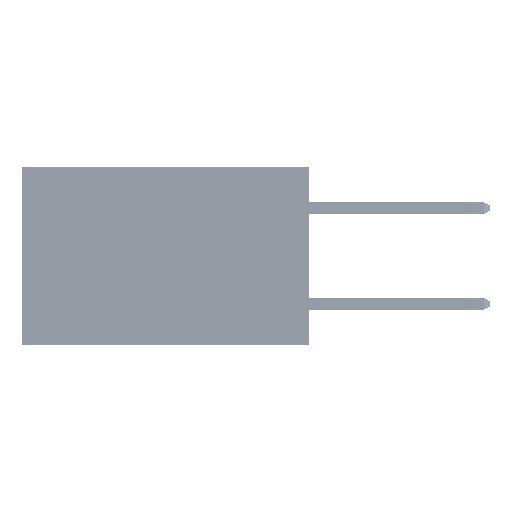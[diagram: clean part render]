
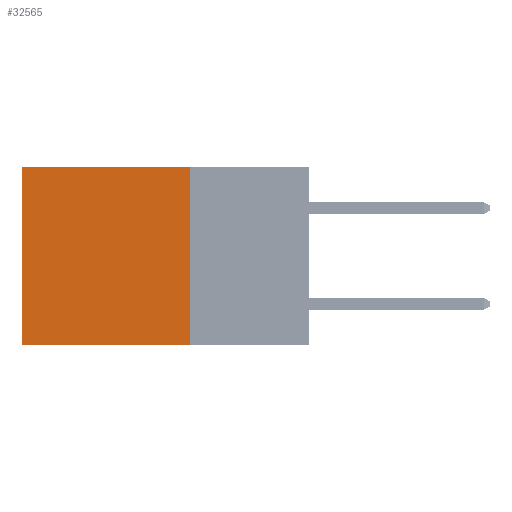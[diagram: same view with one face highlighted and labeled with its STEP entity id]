
A CAD part, left-side view. The second image highlights one B-rep face of the part: STEP entity #32565.
In plain terms, the highlighted planar face has unit normal (-1, 0, 0).
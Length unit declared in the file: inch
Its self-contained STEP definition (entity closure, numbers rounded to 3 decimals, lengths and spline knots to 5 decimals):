
#856 = PLANE ( 'NONE',  #13473 ) ;
#861 = CARTESIAN_POINT ( 'NONE',  ( 0.2875, 0.25, -0.37 ) ) ;
#1019 = ORIENTED_EDGE ( 'NONE', *, *, #51578, .T. ) ;
#1751 = CARTESIAN_POINT ( 'NONE',  ( 0.2875, 0.25, 0. ) ) ;
#2517 = VECTOR ( 'NONE', #15506, 39.37008 ) ;
#5125 = VECTOR ( 'NONE', #17125, 39.37008 ) ;
#6104 = DIRECTION ( 'NONE',  ( 0., 1., 0. ) ) ;
#7245 = EDGE_LOOP ( 'NONE', ( #50774, #39145, #17629, #1019 ) ) ;
#7819 = EDGE_CURVE ( 'NONE', #8032, #37418, #15131, .T. ) ;
#8032 = VERTEX_POINT ( 'NONE', #20796 ) ;
#10239 = VECTOR ( 'NONE', #6104, 39.37008 ) ;
#10594 = CARTESIAN_POINT ( 'NONE',  ( 0.2875, 0.25, -0.37 ) ) ;
#12822 = CARTESIAN_POINT ( 'NONE',  ( 0.2875, 0.25, 0. ) ) ;
#13473 = AXIS2_PLACEMENT_3D ( 'NONE', #21171, #41553, #17296 ) ;
#15131 = LINE ( 'NONE', #39754, #2517 ) ;
#15506 = DIRECTION ( 'NONE',  ( 0., 0., -1. ) ) ;
#15792 = LINE ( 'NONE', #1751, #28513 ) ;
#17125 = DIRECTION ( 'NONE',  ( 0., 1., 0. ) ) ;
#17296 = DIRECTION ( 'NONE',  ( 0., 0., -1. ) ) ;
#17629 = ORIENTED_EDGE ( 'NONE', *, *, #23222, .F. ) ;
#20382 = LINE ( 'NONE', #29794, #10239 ) ;
#20796 = CARTESIAN_POINT ( 'NONE',  ( 0.2875, 0.6, 0. ) ) ;
#21171 = CARTESIAN_POINT ( 'NONE',  ( 0.2875, 0.25, 0. ) ) ;
#23222 = EDGE_CURVE ( 'NONE', #39502, #45514, #15792, .T. ) ;
#26594 = LINE ( 'NONE', #861, #5125 ) ;
#28513 = VECTOR ( 'NONE', #30048, 39.37008 ) ;
#29794 = CARTESIAN_POINT ( 'NONE',  ( 0.2875, 0.25, 0. ) ) ;
#30048 = DIRECTION ( 'NONE',  ( 0., 0., -1. ) ) ;
#32565 = ADVANCED_FACE ( 'NONE', ( #36219 ), #856, .F. ) ;
#36219 = FACE_OUTER_BOUND ( 'NONE', #7245, .T. ) ;
#37418 = VERTEX_POINT ( 'NONE', #49398 ) ;
#39145 = ORIENTED_EDGE ( 'NONE', *, *, #43060, .F. ) ;
#39502 = VERTEX_POINT ( 'NONE', #12822 ) ;
#39754 = CARTESIAN_POINT ( 'NONE',  ( 0.2875, 0.6, 0. ) ) ;
#41553 = DIRECTION ( 'NONE',  ( 1., 0., 0. ) ) ;
#43060 = EDGE_CURVE ( 'NONE', #45514, #37418, #26594, .T. ) ;
#45514 = VERTEX_POINT ( 'NONE', #10594 ) ;
#49398 = CARTESIAN_POINT ( 'NONE',  ( 0.2875, 0.6, -0.37 ) ) ;
#50774 = ORIENTED_EDGE ( 'NONE', *, *, #7819, .T. ) ;
#51578 = EDGE_CURVE ( 'NONE', #39502, #8032, #20382, .T. ) ;
